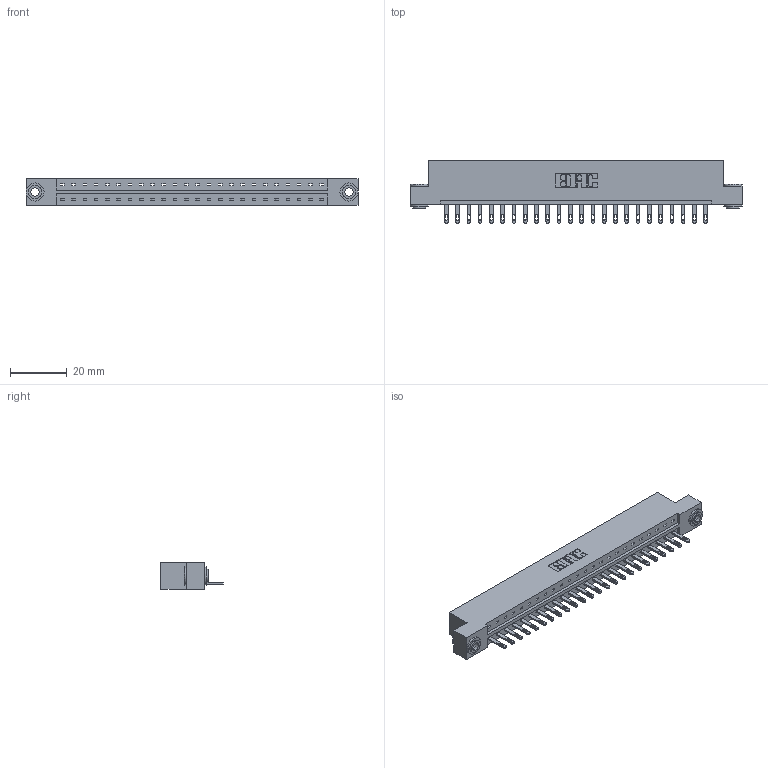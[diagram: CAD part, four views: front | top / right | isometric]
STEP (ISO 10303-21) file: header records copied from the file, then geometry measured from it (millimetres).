
FILE_DESCRIPTION (( 'STEP AP203' ), '1' );
FILE_NAME ('833-024-500-103.STEP', '2020-06-01T19:53:59', ( '' ), ( '' ), 'SwSTEP 2.0', 'SolidWorks 2020', '' );
FILE_SCHEMA (( 'CONFIG_CONTROL_DESIGN' ));
Length unit declared in the file: inch
Products named in the file (4): 345-250-002_345-250-002-102; 345-292-001_345-293-100; 833-024-500-103; 833 Part_Flush - .156 Dia - TH
Assembly tree (27 placements, depth 2):
  833-024-500-103
    833 Part_Flush - .156 Dia - TH
    345-292-001_345-293-100  x24
    345-250-002_345-250-002-102  x2
Bounding box: 116.64 x 21.85 x 9.4 mm (x, y, z)
Volume: 11616.4 mm3; surface area: 12736.8 mm2
Topology: 27 solids, 27 shells, 1448 faces, 4419 edges, 2942 vertices
Faces by surface type: plane 944, cylinder 496, cone 8
Entity records: 17580 total; most frequent: CARTESIAN_POINT 3013, ORIENTED_EDGE 2966, DIRECTION 2613, EDGE_CURVE 1483, VECTOR 1327, LINE 1327, VERTEX_POINT 986, AXIS2_PLACEMENT_3D 643
